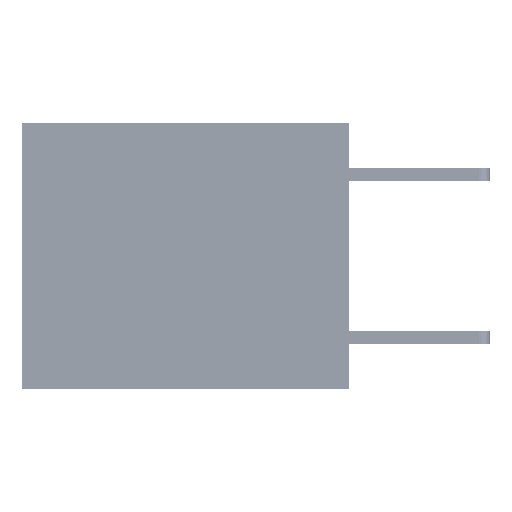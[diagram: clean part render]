
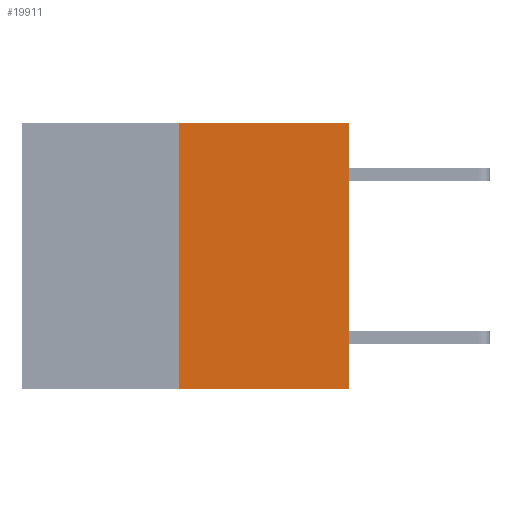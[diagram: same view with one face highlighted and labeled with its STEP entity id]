
A CAD part, left-side view. The second image highlights one B-rep face of the part: STEP entity #19911.
In plain terms, the highlighted planar face has unit normal (-1, 0, 0).
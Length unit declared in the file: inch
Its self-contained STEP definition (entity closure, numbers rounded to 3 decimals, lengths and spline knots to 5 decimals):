
#2397 = DIRECTION ( 'NONE',  ( 1., 0., 0. ) ) ;
#2519 = PLANE ( 'NONE',  #27519 ) ;
#3162 = VECTOR ( 'NONE', #30443, 39.37008 ) ;
#3419 = CARTESIAN_POINT ( 'NONE',  ( 0., 0., -0.49 ) ) ;
#3774 = LINE ( 'NONE', #6645, #24722 ) ;
#5804 = CARTESIAN_POINT ( 'NONE',  ( 0., 0.312, -0.49 ) ) ;
#6645 = CARTESIAN_POINT ( 'NONE',  ( 0., 0.312, -0.49 ) ) ;
#6646 = FACE_OUTER_BOUND ( 'NONE', #13025, .T. ) ;
#7866 = VERTEX_POINT ( 'NONE', #3419 ) ;
#8342 = CARTESIAN_POINT ( 'NONE',  ( 0., 0.6, -0.49 ) ) ;
#9431 = ORIENTED_EDGE ( 'NONE', *, *, #28505, .T. ) ;
#10036 = CARTESIAN_POINT ( 'NONE',  ( 0., 0.312, 0. ) ) ;
#10413 = LINE ( 'NONE', #8342, #3162 ) ;
#13025 = EDGE_LOOP ( 'NONE', ( #32915, #19663, #9431, #20780 ) ) ;
#14182 = DIRECTION ( 'NONE',  ( 0., -1., 0. ) ) ;
#14452 = LINE ( 'NONE', #16826, #30306 ) ;
#16780 = CARTESIAN_POINT ( 'NONE',  ( 0., 0., 0. ) ) ;
#16826 = CARTESIAN_POINT ( 'NONE',  ( 0., 0., 0. ) ) ;
#19243 = DIRECTION ( 'NONE',  ( 0., 0., 1. ) ) ;
#19663 = ORIENTED_EDGE ( 'NONE', *, *, #25517, .T. ) ;
#19911 = ADVANCED_FACE ( 'NONE', ( #6646 ), #2519, .F. ) ;
#20780 = ORIENTED_EDGE ( 'NONE', *, *, #24349, .F. ) ;
#21408 = VERTEX_POINT ( 'NONE', #5804 ) ;
#21623 = CARTESIAN_POINT ( 'NONE',  ( 0., 0.6, 0. ) ) ;
#23198 = EDGE_CURVE ( 'NONE', #21408, #28803, #3774, .T. ) ;
#24349 = EDGE_CURVE ( 'NONE', #28803, #31948, #26749, .T. ) ;
#24722 = VECTOR ( 'NONE', #25832, 39.37008 ) ;
#25517 = EDGE_CURVE ( 'NONE', #21408, #7866, #10413, .T. ) ;
#25832 = DIRECTION ( 'NONE',  ( 0., 0., 1. ) ) ;
#26749 = LINE ( 'NONE', #33479, #34057 ) ;
#27519 = AXIS2_PLACEMENT_3D ( 'NONE', #21623, #2397, #32664 ) ;
#28505 = EDGE_CURVE ( 'NONE', #7866, #31948, #14452, .T. ) ;
#28803 = VERTEX_POINT ( 'NONE', #10036 ) ;
#30306 = VECTOR ( 'NONE', #19243, 39.37008 ) ;
#30443 = DIRECTION ( 'NONE',  ( 0., -1., 0. ) ) ;
#31948 = VERTEX_POINT ( 'NONE', #16780 ) ;
#32664 = DIRECTION ( 'NONE',  ( 0., 0., -1. ) ) ;
#32915 = ORIENTED_EDGE ( 'NONE', *, *, #23198, .F. ) ;
#33479 = CARTESIAN_POINT ( 'NONE',  ( 0., 0.6, 0. ) ) ;
#34057 = VECTOR ( 'NONE', #14182, 39.37008 ) ;
